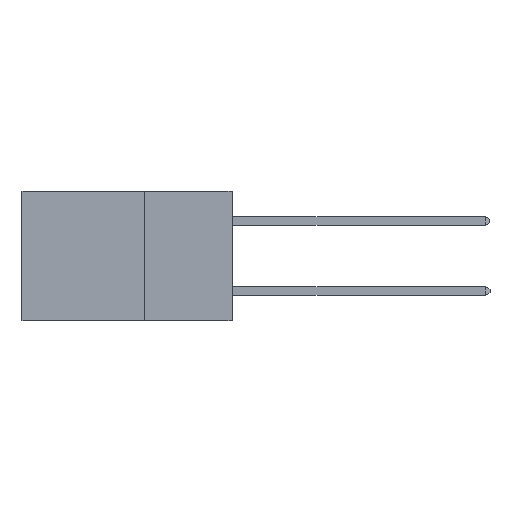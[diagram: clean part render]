
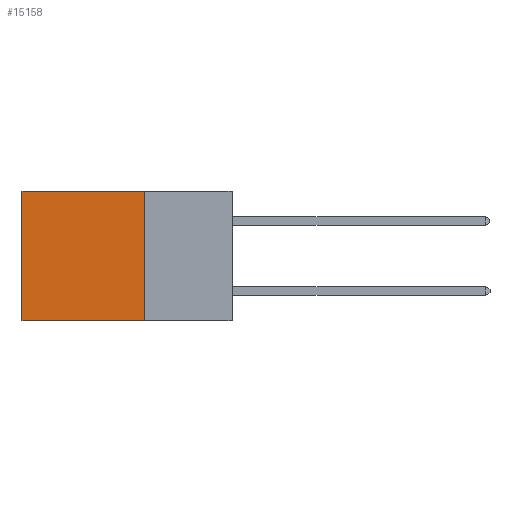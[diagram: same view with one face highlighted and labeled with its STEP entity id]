
A CAD part, left-side view. The second image highlights one B-rep face of the part: STEP entity #15158.
In plain terms, the highlighted planar face has unit normal (-1, 0, 0).
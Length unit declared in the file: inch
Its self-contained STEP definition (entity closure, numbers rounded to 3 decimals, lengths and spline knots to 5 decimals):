
#2319 = DIRECTION ( 'NONE',  ( 0., 0., -1. ) ) ;
#2339 = VERTEX_POINT ( 'NONE', #2453 ) ;
#2453 = CARTESIAN_POINT ( 'NONE',  ( 0.2875, 0.6, -0.37 ) ) ;
#2566 = CARTESIAN_POINT ( 'NONE',  ( 0.2875, 0.25, 0. ) ) ;
#2798 = VERTEX_POINT ( 'NONE', #8081 ) ;
#4384 = CARTESIAN_POINT ( 'NONE',  ( 0.2875, 0.25, -0.37 ) ) ;
#5286 = DIRECTION ( 'NONE',  ( 0., 1., 0. ) ) ;
#5384 = EDGE_LOOP ( 'NONE', ( #17406, #8094, #12286, #16327 ) ) ;
#6289 = VERTEX_POINT ( 'NONE', #4384 ) ;
#6304 = EDGE_CURVE ( 'NONE', #2798, #16676, #21837, .T. ) ;
#6659 = CARTESIAN_POINT ( 'NONE',  ( 0.2875, 0.25, -0.37 ) ) ;
#7501 = EDGE_CURVE ( 'NONE', #16676, #2339, #18455, .T. ) ;
#7900 = LINE ( 'NONE', #8716, #23382 ) ;
#8081 = CARTESIAN_POINT ( 'NONE',  ( 0.2875, 0.25, 0. ) ) ;
#8094 = ORIENTED_EDGE ( 'NONE', *, *, #24388, .F. ) ;
#8252 = PLANE ( 'NONE',  #19919 ) ;
#8632 = DIRECTION ( 'NONE',  ( 0., 0., -1. ) ) ;
#8716 = CARTESIAN_POINT ( 'NONE',  ( 0.2875, 0.25, 0. ) ) ;
#8961 = LINE ( 'NONE', #6659, #20533 ) ;
#12286 = ORIENTED_EDGE ( 'NONE', *, *, #19223, .F. ) ;
#13922 = DIRECTION ( 'NONE',  ( 1., 0., 0. ) ) ;
#15158 = ADVANCED_FACE ( 'NONE', ( #18259 ), #8252, .F. ) ;
#15456 = CARTESIAN_POINT ( 'NONE',  ( 0.2875, 0.6, 0. ) ) ;
#16327 = ORIENTED_EDGE ( 'NONE', *, *, #6304, .T. ) ;
#16676 = VERTEX_POINT ( 'NONE', #22142 ) ;
#17406 = ORIENTED_EDGE ( 'NONE', *, *, #7501, .T. ) ;
#17564 = VECTOR ( 'NONE', #19334, 39.37008 ) ;
#18259 = FACE_OUTER_BOUND ( 'NONE', #5384, .T. ) ;
#18455 = LINE ( 'NONE', #15456, #17564 ) ;
#18583 = CARTESIAN_POINT ( 'NONE',  ( 0.2875, 0.25, 0. ) ) ;
#19223 = EDGE_CURVE ( 'NONE', #2798, #6289, #7900, .T. ) ;
#19334 = DIRECTION ( 'NONE',  ( 0., 0., -1. ) ) ;
#19919 = AXIS2_PLACEMENT_3D ( 'NONE', #2566, #13922, #2319 ) ;
#20196 = DIRECTION ( 'NONE',  ( 0., 1., 0. ) ) ;
#20533 = VECTOR ( 'NONE', #20196, 39.37008 ) ;
#21837 = LINE ( 'NONE', #18583, #23326 ) ;
#22142 = CARTESIAN_POINT ( 'NONE',  ( 0.2875, 0.6, 0. ) ) ;
#23326 = VECTOR ( 'NONE', #5286, 39.37008 ) ;
#23382 = VECTOR ( 'NONE', #8632, 39.37008 ) ;
#24388 = EDGE_CURVE ( 'NONE', #6289, #2339, #8961, .T. ) ;
